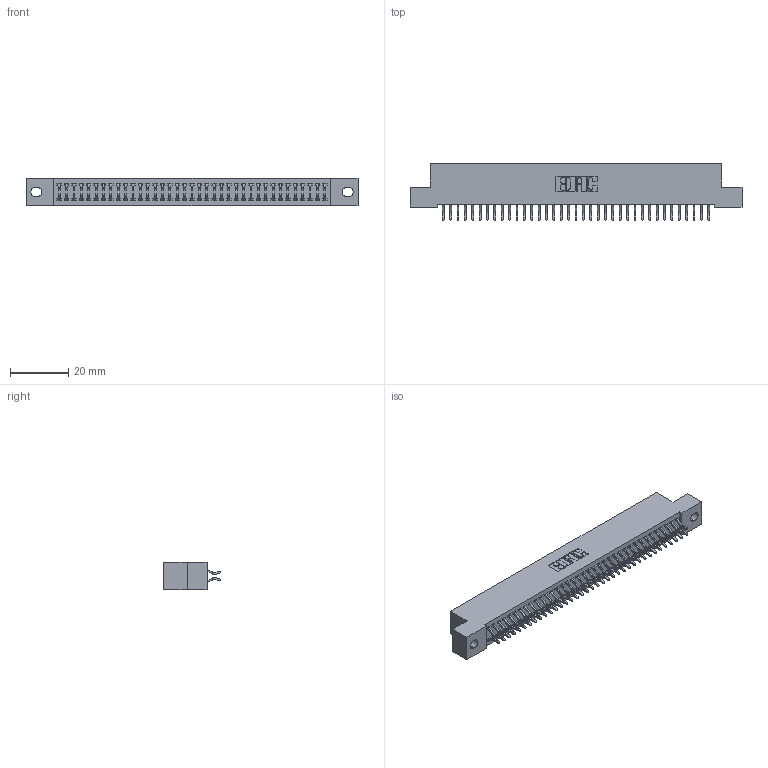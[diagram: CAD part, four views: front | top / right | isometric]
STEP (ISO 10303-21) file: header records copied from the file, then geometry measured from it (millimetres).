
FILE_DESCRIPTION (( 'STEP AP203' ), '1' );
FILE_NAME ('392-074-556-202.STEP', '2018-08-18T00:59:28', ( '' ), ( '' ), 'SwSTEP 2.0', 'SolidWorks 2016', '' );
FILE_SCHEMA (( 'CONFIG_CONTROL_DESIGN' ));
Length unit declared in the file: inch
Products named in the file (3): 345-292-001_556 Tail; 392-074-556-202; 342 Part_.128 Slot
Assembly tree (75 placements, depth 2):
  392-074-556-202
    342 Part_.128 Slot
    345-292-001_556 Tail  x74
Bounding box: 114.3 x 19.58 x 9.4 mm (x, y, z)
Volume: 10192.2 mm3; surface area: 16154.8 mm2
Topology: 75 solids, 75 shells, 4406 faces, 13113 edges, 8642 vertices
Faces by surface type: plane 3030, cylinder 1376
Entity records: 24673 total; most frequent: CARTESIAN_POINT 4110, ORIENTED_EDGE 4034, DIRECTION 3509, EDGE_CURVE 2017, VECTOR 1881, LINE 1881, VERTEX_POINT 1342, AXIS2_PLACEMENT_3D 814
